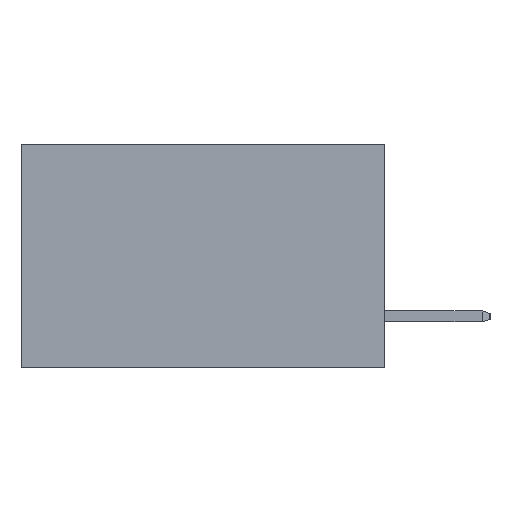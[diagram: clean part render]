
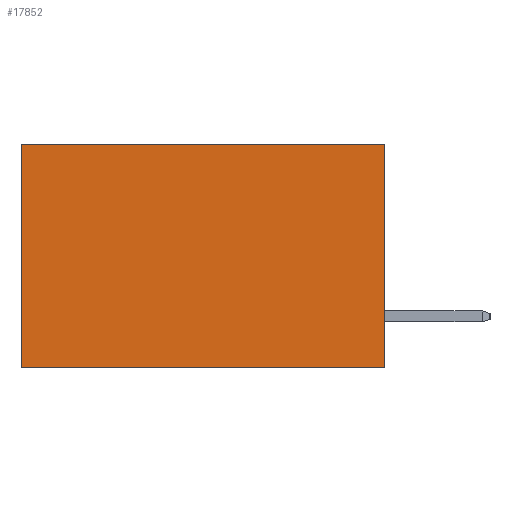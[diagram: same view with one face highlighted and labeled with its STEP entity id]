
A CAD part, left-side view. The second image highlights one B-rep face of the part: STEP entity #17852.
In plain terms, the highlighted planar face has unit normal (-1, 0, 0).
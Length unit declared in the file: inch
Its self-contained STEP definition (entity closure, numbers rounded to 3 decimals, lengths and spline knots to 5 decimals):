
#1476 = AXIS2_PLACEMENT_3D ( 'NONE', #18878, #22874, #11046 ) ;
#1730 = VECTOR ( 'NONE', #19800, 39.37008 ) ;
#1878 = CARTESIAN_POINT ( 'NONE',  ( 0.2615, 0.6, -0.37 ) ) ;
#2469 = DIRECTION ( 'NONE',  ( 0., 0., -1. ) ) ;
#3868 = CARTESIAN_POINT ( 'NONE',  ( 0.2615, 0., 0. ) ) ;
#4396 = CARTESIAN_POINT ( 'NONE',  ( 0.2615, 0.6, -0.37 ) ) ;
#5902 = VECTOR ( 'NONE', #18550, 39.37008 ) ;
#6480 = VERTEX_POINT ( 'NONE', #7054 ) ;
#6533 = LINE ( 'NONE', #21130, #20947 ) ;
#6768 = CARTESIAN_POINT ( 'NONE',  ( 0.2615, 0., -0.37 ) ) ;
#6910 = LINE ( 'NONE', #15834, #1730 ) ;
#7054 = CARTESIAN_POINT ( 'NONE',  ( 0.2615, 0., -0.37 ) ) ;
#8455 = EDGE_CURVE ( 'NONE', #23248, #21815, #19727, .T. ) ;
#9055 = PLANE ( 'NONE',  #1476 ) ;
#9212 = VECTOR ( 'NONE', #2469, 39.37008 ) ;
#11046 = DIRECTION ( 'NONE',  ( 0., 0., -1. ) ) ;
#11748 = ORIENTED_EDGE ( 'NONE', *, *, #14948, .F. ) ;
#12025 = EDGE_LOOP ( 'NONE', ( #19474, #23080, #11748, #24560 ) ) ;
#12574 = EDGE_CURVE ( 'NONE', #14163, #23248, #6533, .T. ) ;
#13044 = EDGE_CURVE ( 'NONE', #6480, #21815, #20924, .T. ) ;
#13316 = DIRECTION ( 'NONE',  ( 0., 1., 0. ) ) ;
#14163 = VERTEX_POINT ( 'NONE', #3868 ) ;
#14197 = FACE_OUTER_BOUND ( 'NONE', #12025, .T. ) ;
#14948 = EDGE_CURVE ( 'NONE', #14163, #6480, #6910, .T. ) ;
#15834 = CARTESIAN_POINT ( 'NONE',  ( 0.2615, 0., -0.37 ) ) ;
#17852 = ADVANCED_FACE ( 'NONE', ( #14197 ), #9055, .F. ) ;
#18550 = DIRECTION ( 'NONE',  ( 0., 1., 0. ) ) ;
#18878 = CARTESIAN_POINT ( 'NONE',  ( 0.2615, 0., -0.37 ) ) ;
#19474 = ORIENTED_EDGE ( 'NONE', *, *, #8455, .T. ) ;
#19727 = LINE ( 'NONE', #4396, #9212 ) ;
#19800 = DIRECTION ( 'NONE',  ( 0., 0., -1. ) ) ;
#20924 = LINE ( 'NONE', #6768, #5902 ) ;
#20947 = VECTOR ( 'NONE', #13316, 39.37008 ) ;
#21130 = CARTESIAN_POINT ( 'NONE',  ( 0.2615, 0., 0. ) ) ;
#21815 = VERTEX_POINT ( 'NONE', #1878 ) ;
#22874 = DIRECTION ( 'NONE',  ( 1., 0., 0. ) ) ;
#23080 = ORIENTED_EDGE ( 'NONE', *, *, #13044, .F. ) ;
#23248 = VERTEX_POINT ( 'NONE', #23488 ) ;
#23488 = CARTESIAN_POINT ( 'NONE',  ( 0.2615, 0.6, 0. ) ) ;
#24560 = ORIENTED_EDGE ( 'NONE', *, *, #12574, .T. ) ;
